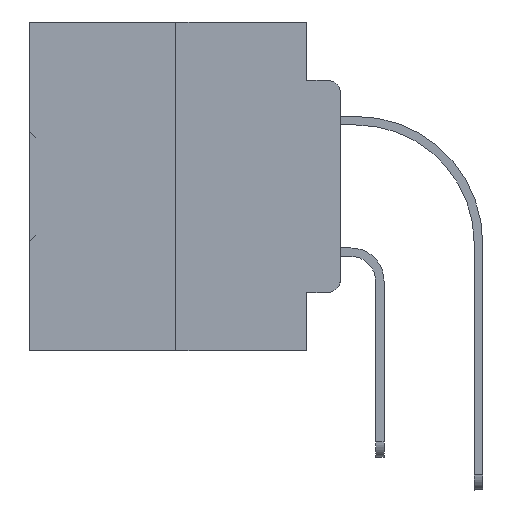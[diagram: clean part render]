
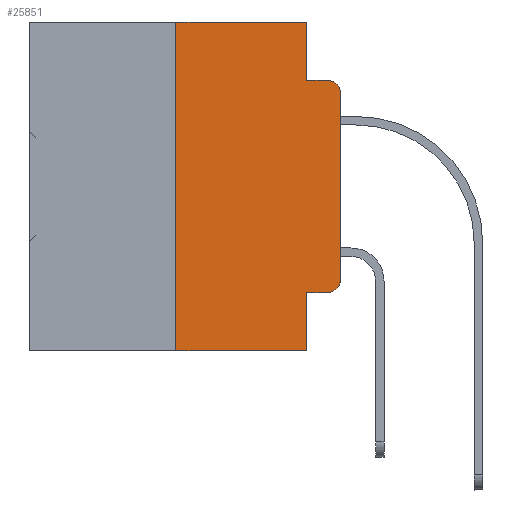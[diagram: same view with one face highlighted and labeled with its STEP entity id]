
A CAD part, left-side view. The second image highlights one B-rep face of the part: STEP entity #25851.
In plain terms, the highlighted planar face has unit normal (-1, 0, 0).
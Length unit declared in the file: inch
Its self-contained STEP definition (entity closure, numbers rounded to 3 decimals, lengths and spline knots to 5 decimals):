
#222 = VERTEX_POINT ( 'NONE', #7119 ) ;
#368 = CARTESIAN_POINT ( 'NONE',  ( 0., 0.051, -0.5 ) ) ;
#565 = CARTESIAN_POINT ( 'NONE',  ( 0., 0.473, -0.5 ) ) ;
#685 = CARTESIAN_POINT ( 'NONE',  ( 0., 0.25, 0. ) ) ;
#1930 = DIRECTION ( 'NONE',  ( 0., -1., 0. ) ) ;
#1971 = CARTESIAN_POINT ( 'NONE',  ( 0., 0.051, -0.0885 ) ) ;
#2192 = CARTESIAN_POINT ( 'NONE',  ( 0., 0.051, 0. ) ) ;
#3100 = AXIS2_PLACEMENT_3D ( 'NONE', #33082, #23646, #14601 ) ;
#4202 = LINE ( 'NONE', #1971, #31494 ) ;
#4304 = VERTEX_POINT ( 'NONE', #368 ) ;
#5090 = ORIENTED_EDGE ( 'NONE', *, *, #5672, .T. ) ;
#5198 = VECTOR ( 'NONE', #24557, 39.37008 ) ;
#5330 = EDGE_CURVE ( 'NONE', #222, #15366, #32269, .T. ) ;
#5672 = EDGE_CURVE ( 'NONE', #6620, #4304, #28025, .T. ) ;
#6620 = VERTEX_POINT ( 'NONE', #35664 ) ;
#6895 = CARTESIAN_POINT ( 'NONE',  ( 0., 0.25, 0. ) ) ;
#7119 = CARTESIAN_POINT ( 'NONE',  ( 0., 0., -0.3915 ) ) ;
#7222 = CARTESIAN_POINT ( 'NONE',  ( 0., 0.051, 0. ) ) ;
#7426 = DIRECTION ( 'NONE',  ( 0., 0., -1. ) ) ;
#7479 = VERTEX_POINT ( 'NONE', #7952 ) ;
#7952 = CARTESIAN_POINT ( 'NONE',  ( 0., 0.051, 0. ) ) ;
#8680 = EDGE_CURVE ( 'NONE', #33183, #29280, #25708, .T. ) ;
#10286 = CARTESIAN_POINT ( 'NONE',  ( 0., 0.02, -0.4115 ) ) ;
#11247 = ORIENTED_EDGE ( 'NONE', *, *, #24411, .T. ) ;
#11320 = CARTESIAN_POINT ( 'NONE',  ( 0., 0.02, -0.3915 ) ) ;
#11500 = DIRECTION ( 'NONE',  ( 0., 0., -1. ) ) ;
#11858 = AXIS2_PLACEMENT_3D ( 'NONE', #17323, #29575, #23959 ) ;
#12407 = CARTESIAN_POINT ( 'NONE',  ( 0., 0., -0.1085 ) ) ;
#14041 = DIRECTION ( 'NONE',  ( 0., -1., 0. ) ) ;
#14601 = DIRECTION ( 'NONE',  ( 0., 0., -1. ) ) ;
#15366 = VERTEX_POINT ( 'NONE', #12407 ) ;
#16747 = VERTEX_POINT ( 'NONE', #23811 ) ;
#16821 = LINE ( 'NONE', #7222, #28392 ) ;
#17013 = DIRECTION ( 'NONE',  ( 0., 0., 1. ) ) ;
#17323 = CARTESIAN_POINT ( 'NONE',  ( 0., 0.02, -0.1085 ) ) ;
#19274 = ORIENTED_EDGE ( 'NONE', *, *, #20179, .T. ) ;
#19820 = DIRECTION ( 'NONE',  ( 0., -1., 0. ) ) ;
#20179 = EDGE_CURVE ( 'NONE', #29280, #222, #36661, .T. ) ;
#20621 = EDGE_CURVE ( 'NONE', #33183, #4304, #16821, .T. ) ;
#21018 = FACE_OUTER_BOUND ( 'NONE', #31886, .T. ) ;
#22737 = CIRCLE ( 'NONE', #11858, 0.02 ) ;
#23624 = DIRECTION ( 'NONE',  ( 0., 0., -1. ) ) ;
#23646 = DIRECTION ( 'NONE',  ( 1., 0., 0. ) ) ;
#23811 = CARTESIAN_POINT ( 'NONE',  ( 0., 0.051, -0.0885 ) ) ;
#23959 = DIRECTION ( 'NONE',  ( 0., 0., -1. ) ) ;
#24411 = EDGE_CURVE ( 'NONE', #15366, #33344, #22737, .T. ) ;
#24557 = DIRECTION ( 'NONE',  ( 0., 0., 1. ) ) ;
#25112 = VECTOR ( 'NONE', #1930, 39.37008 ) ;
#25708 = LINE ( 'NONE', #26709, #35912 ) ;
#25851 = ADVANCED_FACE ( 'NONE', ( #21018 ), #30646, .F. ) ;
#26709 = CARTESIAN_POINT ( 'NONE',  ( 0., 0.051, -0.4115 ) ) ;
#27051 = CARTESIAN_POINT ( 'NONE',  ( 0., 0.051, -0.4115 ) ) ;
#27074 = AXIS2_PLACEMENT_3D ( 'NONE', #11320, #29181, #11500 ) ;
#27285 = VECTOR ( 'NONE', #23624, 39.37008 ) ;
#28025 = LINE ( 'NONE', #565, #25112 ) ;
#28295 = EDGE_CURVE ( 'NONE', #6620, #34253, #31166, .T. ) ;
#28392 = VECTOR ( 'NONE', #7426, 39.37008 ) ;
#29181 = DIRECTION ( 'NONE',  ( -1., 0., 0. ) ) ;
#29280 = VERTEX_POINT ( 'NONE', #10286 ) ;
#29575 = DIRECTION ( 'NONE',  ( -1., 0., 0. ) ) ;
#30330 = VECTOR ( 'NONE', #19820, 39.37008 ) ;
#30540 = ORIENTED_EDGE ( 'NONE', *, *, #33050, .F. ) ;
#30626 = ORIENTED_EDGE ( 'NONE', *, *, #36790, .F. ) ;
#30646 = PLANE ( 'NONE',  #3100 ) ;
#31166 = LINE ( 'NONE', #685, #5198 ) ;
#31230 = ORIENTED_EDGE ( 'NONE', *, *, #8680, .T. ) ;
#31494 = VECTOR ( 'NONE', #34880, 39.37008 ) ;
#31750 = EDGE_CURVE ( 'NONE', #16747, #33344, #4202, .T. ) ;
#31886 = EDGE_LOOP ( 'NONE', ( #35208, #11247, #39016, #30626, #30540, #33933, #5090, #33140, #31230, #19274 ) ) ;
#32269 = LINE ( 'NONE', #38071, #35961 ) ;
#33050 = EDGE_CURVE ( 'NONE', #34253, #7479, #35076, .T. ) ;
#33082 = CARTESIAN_POINT ( 'NONE',  ( 0., 0.473, 0. ) ) ;
#33140 = ORIENTED_EDGE ( 'NONE', *, *, #20621, .F. ) ;
#33183 = VERTEX_POINT ( 'NONE', #27051 ) ;
#33344 = VERTEX_POINT ( 'NONE', #37646 ) ;
#33933 = ORIENTED_EDGE ( 'NONE', *, *, #28295, .F. ) ;
#34253 = VERTEX_POINT ( 'NONE', #6895 ) ;
#34880 = DIRECTION ( 'NONE',  ( 0., -1., 0. ) ) ;
#34891 = CARTESIAN_POINT ( 'NONE',  ( 0., 0.473, 0. ) ) ;
#35076 = LINE ( 'NONE', #34891, #30330 ) ;
#35208 = ORIENTED_EDGE ( 'NONE', *, *, #5330, .T. ) ;
#35664 = CARTESIAN_POINT ( 'NONE',  ( 0., 0.25, -0.5 ) ) ;
#35912 = VECTOR ( 'NONE', #14041, 39.37008 ) ;
#35961 = VECTOR ( 'NONE', #17013, 39.37008 ) ;
#36661 = CIRCLE ( 'NONE', #27074, 0.02 ) ;
#36790 = EDGE_CURVE ( 'NONE', #7479, #16747, #39037, .T. ) ;
#37646 = CARTESIAN_POINT ( 'NONE',  ( 0., 0.02, -0.0885 ) ) ;
#38071 = CARTESIAN_POINT ( 'NONE',  ( 0., 0., 0. ) ) ;
#39016 = ORIENTED_EDGE ( 'NONE', *, *, #31750, .F. ) ;
#39037 = LINE ( 'NONE', #2192, #27285 ) ;
